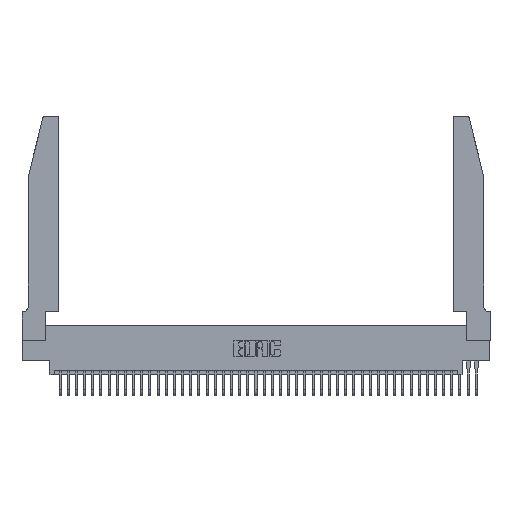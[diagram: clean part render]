
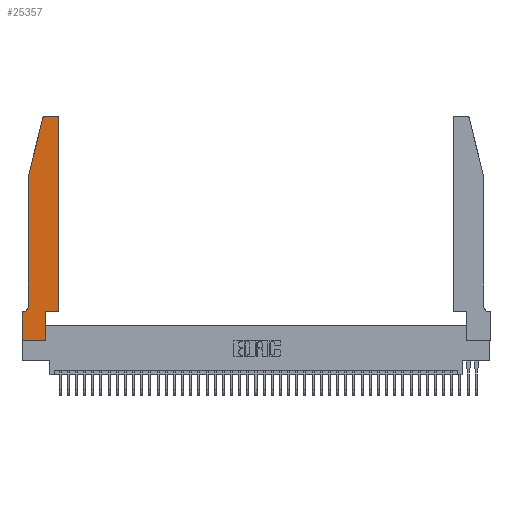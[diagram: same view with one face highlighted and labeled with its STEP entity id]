
A CAD part, top view. The second image highlights one B-rep face of the part: STEP entity #25357.
In plain terms, the highlighted planar face has unit normal (0, 0, 1).
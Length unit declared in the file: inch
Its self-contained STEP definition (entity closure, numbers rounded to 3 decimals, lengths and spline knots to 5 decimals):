
#1363 = VERTEX_POINT ( 'NONE', #23375 ) ;
#1424 = EDGE_CURVE ( 'NONE', #34505, #34053, #18251, .T. ) ;
#1570 = CARTESIAN_POINT ( 'NONE',  ( 0.2865, 0.35, 0.37 ) ) ;
#2226 = CARTESIAN_POINT ( 'NONE',  ( 0.284, 2.72, 0.37 ) ) ;
#3856 = ORIENTED_EDGE ( 'NONE', *, *, #35578, .T. ) ;
#5265 = EDGE_CURVE ( 'NONE', #10357, #31887, #29082, .T. ) ;
#5354 = ORIENTED_EDGE ( 'NONE', *, *, #32317, .T. ) ;
#5570 = AXIS2_PLACEMENT_3D ( 'NONE', #33969, #37061, #18687 ) ;
#5572 = DIRECTION ( 'NONE',  ( 1., 0., 0. ) ) ;
#5681 = CARTESIAN_POINT ( 'NONE',  ( 0.2605, 2.75, 0.37 ) ) ;
#5774 = CARTESIAN_POINT ( 'NONE',  ( 0., 0., 0.37 ) ) ;
#6218 = VERTEX_POINT ( 'NONE', #16798 ) ;
#6974 = LINE ( 'NONE', #25783, #23071 ) ;
#7789 = VERTEX_POINT ( 'NONE', #18506 ) ;
#8603 = VECTOR ( 'NONE', #17621, 39.37008 ) ;
#9828 = CARTESIAN_POINT ( 'NONE',  ( 0.2865, 0.35, 0.37 ) ) ;
#10357 = VERTEX_POINT ( 'NONE', #23360 ) ;
#10492 = ORIENTED_EDGE ( 'NONE', *, *, #28771, .T. ) ;
#11390 = VERTEX_POINT ( 'NONE', #16985 ) ;
#11766 = ORIENTED_EDGE ( 'NONE', *, *, #5265, .T. ) ;
#12200 = PLANE ( 'NONE',  #5570 ) ;
#12539 = VERTEX_POINT ( 'NONE', #23086 ) ;
#13992 = CARTESIAN_POINT ( 'NONE',  ( 0.4505, 0.35, 0.37 ) ) ;
#14217 = CARTESIAN_POINT ( 'NONE',  ( 0.0755, 2., 0.37 ) ) ;
#14476 = ORIENTED_EDGE ( 'NONE', *, *, #17583, .T. ) ;
#14925 = ORIENTED_EDGE ( 'NONE', *, *, #19484, .T. ) ;
#15707 = VECTOR ( 'NONE', #31513, 39.37008 ) ;
#16146 = VECTOR ( 'NONE', #24113, 39.37008 ) ;
#16514 = ORIENTED_EDGE ( 'NONE', *, *, #1424, .T. ) ;
#16798 = CARTESIAN_POINT ( 'NONE',  ( 0.4205, 2.75, 0.37 ) ) ;
#16985 = CARTESIAN_POINT ( 'NONE',  ( 0.0755, 2., 0.37 ) ) ;
#17000 = LINE ( 'NONE', #9828, #40635 ) ;
#17043 = ORIENTED_EDGE ( 'NONE', *, *, #20276, .T. ) ;
#17244 = DIRECTION ( 'NONE',  ( 0., 0., -1. ) ) ;
#17469 = DIRECTION ( 'NONE',  ( -0.239, -0.971, 0. ) ) ;
#17583 = EDGE_CURVE ( 'NONE', #7789, #20458, #6974, .T. ) ;
#17621 = DIRECTION ( 'NONE',  ( 1., 0., 0. ) ) ;
#17787 = CARTESIAN_POINT ( 'NONE',  ( 0.4205, 2.72, 0.37 ) ) ;
#18019 = VECTOR ( 'NONE', #37700, 39.37008 ) ;
#18251 = LINE ( 'NONE', #32964, #8603 ) ;
#18506 = CARTESIAN_POINT ( 'NONE',  ( 0.0055, 0.35, 0.37 ) ) ;
#18687 = DIRECTION ( 'NONE',  ( 1., 0., 0. ) ) ;
#19116 = VERTEX_POINT ( 'NONE', #1570 ) ;
#19309 = CARTESIAN_POINT ( 'NONE',  ( 0.4505, 0.35, 0.37 ) ) ;
#19484 = EDGE_CURVE ( 'NONE', #20458, #34505, #26247, .T. ) ;
#20275 = ORIENTED_EDGE ( 'NONE', *, *, #34073, .T. ) ;
#20276 = EDGE_CURVE ( 'NONE', #34053, #19116, #17000, .T. ) ;
#20383 = CARTESIAN_POINT ( 'NONE',  ( 0., 0.35, 0.37 ) ) ;
#20458 = VERTEX_POINT ( 'NONE', #20383 ) ;
#20990 = DIRECTION ( 'NONE',  ( 1., 0., 0. ) ) ;
#21418 = LINE ( 'NONE', #5681, #22383 ) ;
#22383 = VECTOR ( 'NONE', #37151, 39.37008 ) ;
#22697 = DIRECTION ( 'NONE',  ( 0., 1., 0. ) ) ;
#22712 = ORIENTED_EDGE ( 'NONE', *, *, #25174, .T. ) ;
#22713 = DIRECTION ( 'NONE',  ( -1., 0., 0. ) ) ;
#22776 = VECTOR ( 'NONE', #17469, 39.37008 ) ;
#23071 = VECTOR ( 'NONE', #22713, 39.37008 ) ;
#23086 = CARTESIAN_POINT ( 'NONE',  ( 0.0755, 0.42, 0.37 ) ) ;
#23360 = CARTESIAN_POINT ( 'NONE',  ( 0.284, 2.75, 0.37 ) ) ;
#23375 = CARTESIAN_POINT ( 'NONE',  ( 0.4505, 2.72, 0.37 ) ) ;
#23727 = LINE ( 'NONE', #14217, #22776 ) ;
#24113 = DIRECTION ( 'NONE',  ( 0., -1., 0. ) ) ;
#24797 = DIRECTION ( 'NONE',  ( 0., 0., 1. ) ) ;
#24928 = CIRCLE ( 'NONE', #34923, 0.03 ) ;
#25174 = EDGE_CURVE ( 'NONE', #19116, #31634, #30618, .T. ) ;
#25357 = ADVANCED_FACE ( 'NONE', ( #40216 ), #12200, .T. ) ;
#25705 = AXIS2_PLACEMENT_3D ( 'NONE', #2226, #24797, #5572 ) ;
#25783 = CARTESIAN_POINT ( 'NONE',  ( 0.0755, 0.35, 0.37 ) ) ;
#25947 = AXIS2_PLACEMENT_3D ( 'NONE', #35655, #17244, #38799 ) ;
#26205 = CARTESIAN_POINT ( 'NONE',  ( 0.4505, 0.35, 0.37 ) ) ;
#26247 = LINE ( 'NONE', #33919, #18019 ) ;
#28033 = ORIENTED_EDGE ( 'NONE', *, *, #37744, .T. ) ;
#28771 = EDGE_CURVE ( 'NONE', #11390, #12539, #40785, .T. ) ;
#29082 = CIRCLE ( 'NONE', #25705, 0.03 ) ;
#29261 = DIRECTION ( 'NONE',  ( 1., 0., 0. ) ) ;
#29470 = EDGE_CURVE ( 'NONE', #1363, #6218, #24928, .T. ) ;
#30618 = LINE ( 'NONE', #26205, #37807 ) ;
#31513 = DIRECTION ( 'NONE',  ( 0., 1., 0. ) ) ;
#31634 = VERTEX_POINT ( 'NONE', #13992 ) ;
#31887 = VERTEX_POINT ( 'NONE', #33920 ) ;
#32185 = LINE ( 'NONE', #19309, #15707 ) ;
#32317 = EDGE_CURVE ( 'NONE', #31887, #11390, #23727, .T. ) ;
#32964 = CARTESIAN_POINT ( 'NONE',  ( 0., 0., 0.37 ) ) ;
#33919 = CARTESIAN_POINT ( 'NONE',  ( 0., 0., 0.37 ) ) ;
#33920 = CARTESIAN_POINT ( 'NONE',  ( 0.25487, 2.72718, 0.37 ) ) ;
#33969 = CARTESIAN_POINT ( 'NONE',  ( 0., 0.35, 0.37 ) ) ;
#34053 = VERTEX_POINT ( 'NONE', #37533 ) ;
#34073 = EDGE_CURVE ( 'NONE', #31634, #1363, #32185, .T. ) ;
#34505 = VERTEX_POINT ( 'NONE', #5774 ) ;
#34923 = AXIS2_PLACEMENT_3D ( 'NONE', #17787, #39313, #20990 ) ;
#35578 = EDGE_CURVE ( 'NONE', #12539, #7789, #39288, .T. ) ;
#35655 = CARTESIAN_POINT ( 'NONE',  ( 0.0055, 0.42, 0.37 ) ) ;
#36230 = CARTESIAN_POINT ( 'NONE',  ( 0.0755, 2., 0.37 ) ) ;
#37061 = DIRECTION ( 'NONE',  ( 0., 0., 1. ) ) ;
#37151 = DIRECTION ( 'NONE',  ( -1., 0., 0. ) ) ;
#37331 = ORIENTED_EDGE ( 'NONE', *, *, #29470, .T. ) ;
#37533 = CARTESIAN_POINT ( 'NONE',  ( 0.2865, 0., 0.37 ) ) ;
#37700 = DIRECTION ( 'NONE',  ( 0., -1., 0. ) ) ;
#37744 = EDGE_CURVE ( 'NONE', #6218, #10357, #21418, .T. ) ;
#37807 = VECTOR ( 'NONE', #29261, 39.37008 ) ;
#38774 = EDGE_LOOP ( 'NONE', ( #28033, #11766, #5354, #10492, #3856, #14476, #14925, #16514, #17043, #22712, #20275, #37331 ) ) ;
#38799 = DIRECTION ( 'NONE',  ( -1., 0., 0. ) ) ;
#39288 = CIRCLE ( 'NONE', #25947, 0.07 ) ;
#39313 = DIRECTION ( 'NONE',  ( 0., 0., 1. ) ) ;
#40216 = FACE_OUTER_BOUND ( 'NONE', #38774, .T. ) ;
#40635 = VECTOR ( 'NONE', #22697, 39.37008 ) ;
#40785 = LINE ( 'NONE', #36230, #16146 ) ;
